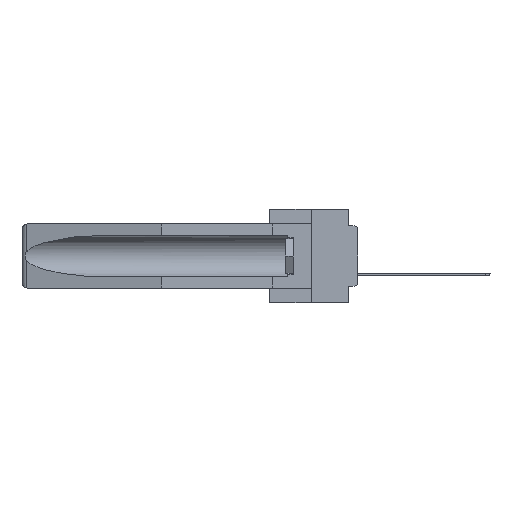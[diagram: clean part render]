
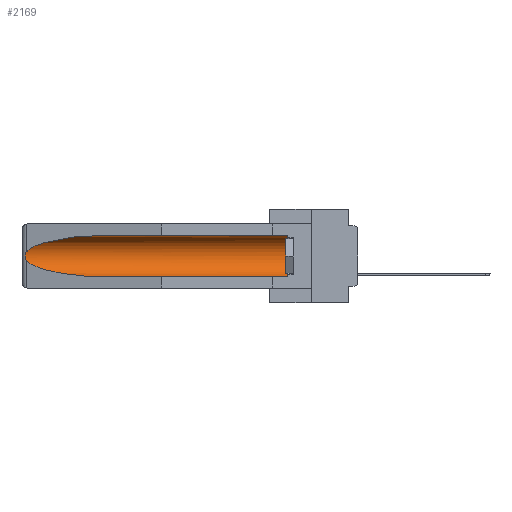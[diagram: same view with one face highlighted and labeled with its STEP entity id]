
A CAD part, left-side view. The second image highlights one B-rep face of the part: STEP entity #2169.
In plain terms, the highlighted cylindrical face has radius 2.857 mm (diameter 5.715 mm), a partial arc.
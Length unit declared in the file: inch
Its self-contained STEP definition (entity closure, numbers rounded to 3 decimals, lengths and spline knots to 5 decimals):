
#981 = VERTEX_POINT ( 'NONE', #20645 ) ;
#1080 = CARTESIAN_POINT ( 'NONE',  ( 0.155, 0.126, -0.284 ) ) ;
#2169 = ADVANCED_FACE ( 'NONE', ( #7774 ), #17844, .F. ) ;
#2801 = DIRECTION ( 'NONE',  ( 0., 1., 0. ) ) ;
#3395 = EDGE_CURVE ( 'NONE', #981, #4663, #19798, .T. ) ;
#3670 = VERTEX_POINT ( 'NONE', #23534 ) ;
#4663 = VERTEX_POINT ( 'NONE', #26731 ) ;
#4773 = CARTESIAN_POINT ( 'NONE',  ( 0.155, -0.30754, -0.059 ) ) ;
#5189 = VERTEX_POINT ( 'NONE', #16397 ) ;
#6165 = CARTESIAN_POINT ( 'NONE',  ( 0.26597, 1.52961, -0.15275 ) ) ;
#6421 = ORIENTED_EDGE ( 'NONE', *, *, #3395, .T. ) ;
#6513 = VERTEX_POINT ( 'NONE', #1080 ) ;
#6877 = EDGE_CURVE ( 'NONE', #3670, #981, #15270, .T. ) ;
#6934 = CARTESIAN_POINT ( 'NONE',  ( 0.26654, 1.53092, -0.15636 ) ) ;
#7066 = ORIENTED_EDGE ( 'NONE', *, *, #22120, .T. ) ;
#7774 = FACE_OUTER_BOUND ( 'NONE', #31333, .T. ) ;
#7941 = CARTESIAN_POINT ( 'NONE',  ( 0.155, -0.30754, -0.1715 ) ) ;
#8123 = DIRECTION ( 'NONE',  ( 0., 0., 1. ) ) ;
#8273 = CARTESIAN_POINT ( 'NONE',  ( 0.26537, 1.52718, -0.19328 ) ) ;
#8386 = AXIS2_PLACEMENT_3D ( 'NONE', #7941, #20485, #20155 ) ;
#8464 = AXIS2_PLACEMENT_3D ( 'NONE', #20664, #15555, #8123 ) ;
#8467 = CARTESIAN_POINT ( 'NONE',  ( 0.26537, 1.52718, -0.14972 ) ) ;
#8966 = CIRCLE ( 'NONE', #8464, 0.1125 ) ;
#9396 = CARTESIAN_POINT ( 'NONE',  ( 0.21114, 1.30732, -0.284 ) ) ;
#11412 = CARTESIAN_POINT ( 'NONE',  ( 0.155, 1.07973, -0.059 ) ) ;
#13262 = EDGE_CURVE ( 'NONE', #6513, #4663, #26470, .T. ) ;
#13741 = CARTESIAN_POINT ( 'NONE',  ( 0.25451, 1.48313, -0.09465 ) ) ;
#13917 = CARTESIAN_POINT ( 'NONE',  ( 0.2673, 1.53269, -0.17917 ) ) ;
#15270 = B_SPLINE_CURVE_WITH_KNOTS ( 'NONE', 3,
 ( #26082, #6165, #6934, #21481, #28388, #23447, #13917, #23617, #28702, #21174 ),
 .UNSPECIFIED., .F., .F.,
 ( 4, 2, 2, 2, 4 ),
 ( 0., 0.00029, 0.00058, 0.00087, 0.00117 ),
 .UNSPECIFIED. ) ;
#15346 = LINE ( 'NONE', #4773, #26171 ) ;
#15555 = DIRECTION ( 'NONE',  ( 0., -1., 0. ) ) ;
#16389 = CARTESIAN_POINT ( 'NONE',  ( 0.21114, 1.30732, -0.059 ) ) ;
#16397 = CARTESIAN_POINT ( 'NONE',  ( 0.155, 1.07973, -0.059 ) ) ;
#17509 =( BOUNDED_CURVE ( )  B_SPLINE_CURVE ( 3, ( #11412, #16389, #13741, #8467 ),
 .UNSPECIFIED., .F., .F. ) 
 B_SPLINE_CURVE_WITH_KNOTS ( ( 4, 4 ),
 ( 4.71239, 6.08839 ),
 .UNSPECIFIED. ) 
 CURVE ( )  GEOMETRIC_REPRESENTATION_ITEM ( )  RATIONAL_B_SPLINE_CURVE ( ( 1., 0.848, 0.848, 1. ) ) 
 REPRESENTATION_ITEM ( '' )  );
#17844 = CYLINDRICAL_SURFACE ( 'NONE', #8386, 0.1125 ) ;
#18863 = VECTOR ( 'NONE', #19574, 39.37008 ) ;
#19574 = DIRECTION ( 'NONE',  ( 0., 1., 0. ) ) ;
#19798 =( BOUNDED_CURVE ( )  B_SPLINE_CURVE ( 3, ( #8273, #26848, #9396, #21609 ),
 .UNSPECIFIED., .F., .F. ) 
 B_SPLINE_CURVE_WITH_KNOTS ( ( 4, 4 ),
 ( 0.1948, 1.5708 ),
 .UNSPECIFIED. ) 
 CURVE ( )  GEOMETRIC_REPRESENTATION_ITEM ( )  RATIONAL_B_SPLINE_CURVE ( ( 1., 0.848, 0.848, 1. ) ) 
 REPRESENTATION_ITEM ( '' )  );
#20155 = DIRECTION ( 'NONE',  ( 0., 0., 1. ) ) ;
#20216 = CARTESIAN_POINT ( 'NONE',  ( 0.155, 0.126, -0.059 ) ) ;
#20485 = DIRECTION ( 'NONE',  ( 0., 1., 0. ) ) ;
#20645 = CARTESIAN_POINT ( 'NONE',  ( 0.26537, 1.52718, -0.19328 ) ) ;
#20664 = CARTESIAN_POINT ( 'NONE',  ( 0.155, 0.126, -0.1715 ) ) ;
#21174 = CARTESIAN_POINT ( 'NONE',  ( 0.26537, 1.52718, -0.19328 ) ) ;
#21481 = CARTESIAN_POINT ( 'NONE',  ( 0.2673, 1.5327, -0.16383 ) ) ;
#21609 = CARTESIAN_POINT ( 'NONE',  ( 0.155, 1.07973, -0.284 ) ) ;
#21858 = CARTESIAN_POINT ( 'NONE',  ( 0.155, -0.30754, -0.284 ) ) ;
#22120 = EDGE_CURVE ( 'NONE', #5189, #3670, #17509, .T. ) ;
#22606 = ORIENTED_EDGE ( 'NONE', *, *, #26775, .T. ) ;
#23447 = CARTESIAN_POINT ( 'NONE',  ( 0.2675, 1.53308, -0.17534 ) ) ;
#23534 = CARTESIAN_POINT ( 'NONE',  ( 0.26537, 1.52718, -0.14972 ) ) ;
#23603 = ORIENTED_EDGE ( 'NONE', *, *, #13262, .F. ) ;
#23617 = CARTESIAN_POINT ( 'NONE',  ( 0.26655, 1.53094, -0.18657 ) ) ;
#26082 = CARTESIAN_POINT ( 'NONE',  ( 0.26537, 1.52718, -0.14972 ) ) ;
#26171 = VECTOR ( 'NONE', #2801, 39.37008 ) ;
#26470 = LINE ( 'NONE', #21858, #18863 ) ;
#26731 = CARTESIAN_POINT ( 'NONE',  ( 0.155, 1.07973, -0.284 ) ) ;
#26775 = EDGE_CURVE ( 'NONE', #30337, #5189, #15346, .T. ) ;
#26848 = CARTESIAN_POINT ( 'NONE',  ( 0.25451, 1.48313, -0.24835 ) ) ;
#27301 = ORIENTED_EDGE ( 'NONE', *, *, #6877, .T. ) ;
#28388 = CARTESIAN_POINT ( 'NONE',  ( 0.2675, 1.53308, -0.16763 ) ) ;
#28702 = CARTESIAN_POINT ( 'NONE',  ( 0.26597, 1.5296, -0.19026 ) ) ;
#29382 = EDGE_CURVE ( 'NONE', #6513, #30337, #8966, .T. ) ;
#30337 = VERTEX_POINT ( 'NONE', #20216 ) ;
#30968 = ORIENTED_EDGE ( 'NONE', *, *, #29382, .T. ) ;
#31333 = EDGE_LOOP ( 'NONE', ( #7066, #27301, #6421, #23603, #30968, #22606 ) ) ;
